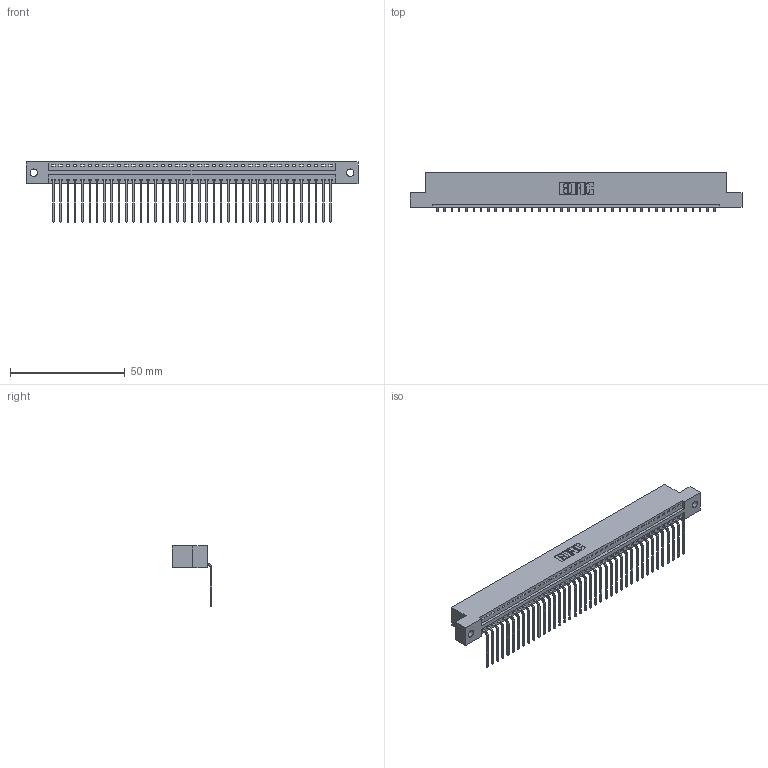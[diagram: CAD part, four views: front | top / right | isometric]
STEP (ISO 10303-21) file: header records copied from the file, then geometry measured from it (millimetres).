
FILE_DESCRIPTION (( 'STEP AP203' ), '1' );
FILE_NAME ('396-039-559-102.STEP', '2019-10-31T22:37:25', ( '' ), ( '' ), 'SwSTEP 2.0', 'SolidWorks 2016', '' );
FILE_SCHEMA (( 'CONFIG_CONTROL_DESIGN' ));
Length unit declared in the file: inch
Products named in the file (3): 346 Part_Flush Mounting Lugs - 0.128 Dia; 345-292-001_558 559 Tail - 1; 396-039-559-102
Assembly tree (40 placements, depth 2):
  396-039-559-102
    346 Part_Flush Mounting Lugs - 0.128 Dia
    345-292-001_558 559 Tail - 1  x39
Bounding box: 144.4 x 17.08 x 26.16 mm (x, y, z)
Volume: 13894.8 mm3; surface area: 17838.2 mm2
Topology: 40 solids, 40 shells, 2462 faces, 7427 edges, 4898 vertices
Faces by surface type: plane 1714, cylinder 748
Entity records: 24695 total; most frequent: CARTESIAN_POINT 4241, ORIENTED_EDGE 4214, DIRECTION 3745, EDGE_CURVE 2107, VECTOR 1819, LINE 1819, VERTEX_POINT 1402, AXIS2_PLACEMENT_3D 963
